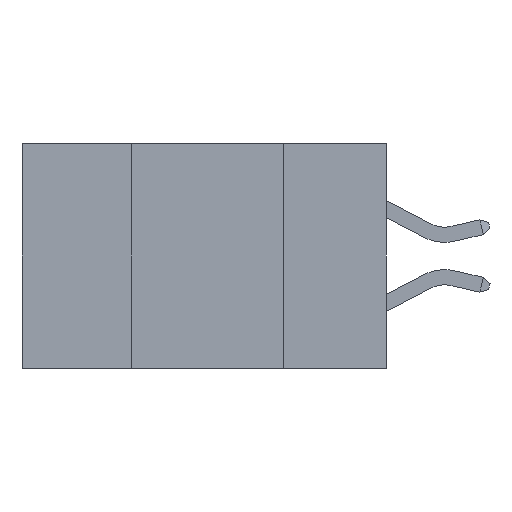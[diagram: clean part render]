
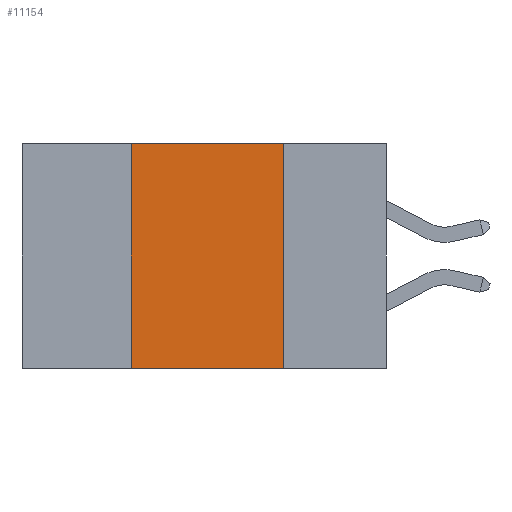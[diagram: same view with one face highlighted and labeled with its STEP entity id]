
A CAD part, left-side view. The second image highlights one B-rep face of the part: STEP entity #11154.
In plain terms, the highlighted planar face has unit normal (-1, 0, 0).
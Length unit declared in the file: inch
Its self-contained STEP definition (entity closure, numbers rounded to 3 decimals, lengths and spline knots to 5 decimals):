
#115 = VERTEX_POINT ( 'NONE', #12250 ) ;
#361 = DIRECTION ( 'NONE',  ( 0., 0., -1. ) ) ;
#1701 = VERTEX_POINT ( 'NONE', #6346 ) ;
#1886 = CARTESIAN_POINT ( 'NONE',  ( 0., 0.6, 0. ) ) ;
#2761 = CARTESIAN_POINT ( 'NONE',  ( 0., 0.42, 0. ) ) ;
#4833 = LINE ( 'NONE', #1886, #14954 ) ;
#5257 = EDGE_LOOP ( 'NONE', ( #7946, #7131, #6624, #5457 ) ) ;
#5457 = ORIENTED_EDGE ( 'NONE', *, *, #22821, .T. ) ;
#6346 = CARTESIAN_POINT ( 'NONE',  ( 0., 0.42, -0.37 ) ) ;
#6624 = ORIENTED_EDGE ( 'NONE', *, *, #15355, .F. ) ;
#7026 = CARTESIAN_POINT ( 'NONE',  ( 0., 0.17, -0.37 ) ) ;
#7131 = ORIENTED_EDGE ( 'NONE', *, *, #9057, .F. ) ;
#7946 = ORIENTED_EDGE ( 'NONE', *, *, #23973, .F. ) ;
#9057 = EDGE_CURVE ( 'NONE', #23228, #115, #4833, .T. ) ;
#9300 = CARTESIAN_POINT ( 'NONE',  ( 0., 0.6, -0.37 ) ) ;
#9671 = VECTOR ( 'NONE', #18567, 39.37008 ) ;
#10048 = CARTESIAN_POINT ( 'NONE',  ( 0., 0.6, 0. ) ) ;
#10145 = CARTESIAN_POINT ( 'NONE',  ( 0., 0.17, -0.37 ) ) ;
#11096 = FACE_OUTER_BOUND ( 'NONE', #5257, .T. ) ;
#11154 = ADVANCED_FACE ( 'NONE', ( #11096 ), #21093, .F. ) ;
#11208 = VECTOR ( 'NONE', #18233, 39.37008 ) ;
#11971 = DIRECTION ( 'NONE',  ( 1., 0., 0. ) ) ;
#12250 = CARTESIAN_POINT ( 'NONE',  ( 0., 0.17, 0. ) ) ;
#13446 = DIRECTION ( 'NONE',  ( 0., -1., 0. ) ) ;
#13476 = LINE ( 'NONE', #18206, #23729 ) ;
#14691 = LINE ( 'NONE', #9300, #9671 ) ;
#14954 = VECTOR ( 'NONE', #13446, 39.37008 ) ;
#15355 = EDGE_CURVE ( 'NONE', #1701, #23228, #13476, .T. ) ;
#16126 = LINE ( 'NONE', #7026, #11208 ) ;
#18206 = CARTESIAN_POINT ( 'NONE',  ( 0., 0.42, -0.37 ) ) ;
#18233 = DIRECTION ( 'NONE',  ( 0., 0., -1. ) ) ;
#18532 = AXIS2_PLACEMENT_3D ( 'NONE', #10048, #11971, #361 ) ;
#18567 = DIRECTION ( 'NONE',  ( 0., -1., 0. ) ) ;
#20026 = DIRECTION ( 'NONE',  ( 0., 0., 1. ) ) ;
#20517 = VERTEX_POINT ( 'NONE', #10145 ) ;
#21093 = PLANE ( 'NONE',  #18532 ) ;
#22821 = EDGE_CURVE ( 'NONE', #1701, #20517, #14691, .T. ) ;
#23228 = VERTEX_POINT ( 'NONE', #2761 ) ;
#23729 = VECTOR ( 'NONE', #20026, 39.37008 ) ;
#23973 = EDGE_CURVE ( 'NONE', #115, #20517, #16126, .T. ) ;
